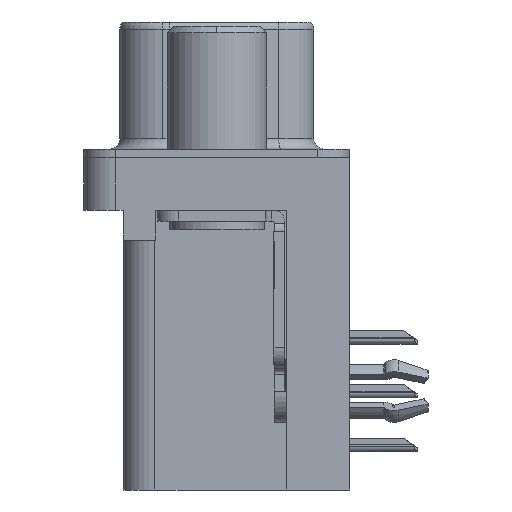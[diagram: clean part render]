
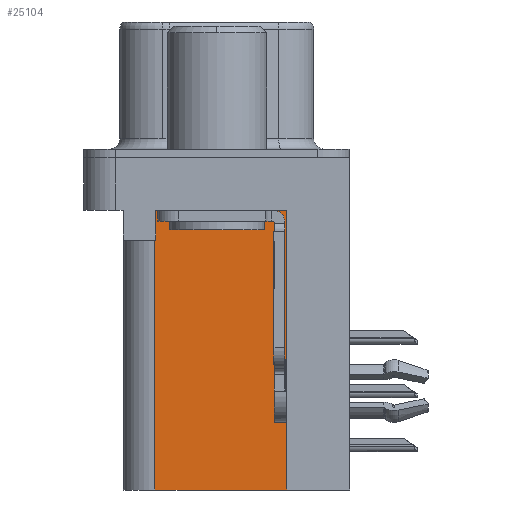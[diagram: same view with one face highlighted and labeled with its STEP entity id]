
A CAD part, left-side view. The second image highlights one B-rep face of the part: STEP entity #25104.
In plain terms, the highlighted planar face has unit normal (-1, 0, 0).
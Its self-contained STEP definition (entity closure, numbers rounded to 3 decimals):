
#221 = ORIENTED_EDGE ( 'NONE', *, *, #28423, .T. ) ;
#751 = VERTEX_POINT ( 'NONE', #20464 ) ;
#1401 = ORIENTED_EDGE ( 'NONE', *, *, #23265, .T. ) ;
#1830 = LINE ( 'NONE', #17029, #31640 ) ;
#3421 = CARTESIAN_POINT ( 'NONE',  ( 3.79, 2.925, -15.7 ) ) ;
#4382 = VERTEX_POINT ( 'NONE', #11301 ) ;
#4682 = DIRECTION ( 'NONE',  ( 0., 0., 1. ) ) ;
#5003 = VECTOR ( 'NONE', #7227, 1000. ) ;
#5517 = CARTESIAN_POINT ( 'NONE',  ( 3.79, 2.895, -3.9 ) ) ;
#5642 = DIRECTION ( 'NONE',  ( 0., 0., -1. ) ) ;
#7227 = DIRECTION ( 'NONE',  ( 0., 1., 0. ) ) ;
#8448 = VERTEX_POINT ( 'NONE', #3421 ) ;
#9052 = ORIENTED_EDGE ( 'NONE', *, *, #11153, .T. ) ;
#9829 = CARTESIAN_POINT ( 'NONE',  ( 3.79, -3.295, -2.5 ) ) ;
#9920 = VERTEX_POINT ( 'NONE', #9829 ) ;
#10063 = ORIENTED_EDGE ( 'NONE', *, *, #30349, .F. ) ;
#11153 = EDGE_CURVE ( 'NONE', #20667, #4382, #27150, .T. ) ;
#11301 = CARTESIAN_POINT ( 'NONE',  ( 3.79, 2.925, -3.9 ) ) ;
#11410 = VECTOR ( 'NONE', #4682, 1000. ) ;
#11549 = AXIS2_PLACEMENT_3D ( 'NONE', #33708, #36646, #19362 ) ;
#12090 = VECTOR ( 'NONE', #14175, 1000. ) ;
#13230 = EDGE_LOOP ( 'NONE', ( #1401, #23926, #9052, #16530, #10063, #221 ) ) ;
#13556 = PLANE ( 'NONE',  #11549 ) ;
#14175 = DIRECTION ( 'NONE',  ( 0., 0., 1. ) ) ;
#14197 = EDGE_CURVE ( 'NONE', #8448, #4382, #28330, .T. ) ;
#15445 = CARTESIAN_POINT ( 'NONE',  ( 3.79, -3.295, -2.5 ) ) ;
#16207 = CARTESIAN_POINT ( 'NONE',  ( 3.79, -3.295, -15.7 ) ) ;
#16530 = ORIENTED_EDGE ( 'NONE', *, *, #14197, .F. ) ;
#16714 = VECTOR ( 'NONE', #5642, 1000. ) ;
#17029 = CARTESIAN_POINT ( 'NONE',  ( 3.79, -3.295, -15.7 ) ) ;
#19362 = DIRECTION ( 'NONE',  ( 0., 0., -1. ) ) ;
#19970 = CARTESIAN_POINT ( 'NONE',  ( 3.79, 2.925, -15.7 ) ) ;
#20464 = CARTESIAN_POINT ( 'NONE',  ( 3.79, 2.895, -2.5 ) ) ;
#20667 = VERTEX_POINT ( 'NONE', #5517 ) ;
#22508 = FACE_OUTER_BOUND ( 'NONE', #13230, .T. ) ;
#23265 = EDGE_CURVE ( 'NONE', #9920, #751, #30709, .T. ) ;
#23926 = ORIENTED_EDGE ( 'NONE', *, *, #23981, .T. ) ;
#23981 = EDGE_CURVE ( 'NONE', #751, #20667, #32036, .T. ) ;
#24518 = VERTEX_POINT ( 'NONE', #25461 ) ;
#24527 = CARTESIAN_POINT ( 'NONE',  ( 3.79, 0., -3.9 ) ) ;
#25104 = ADVANCED_FACE ( 'NONE', ( #22508 ), #13556, .F. ) ;
#25461 = CARTESIAN_POINT ( 'NONE',  ( 3.79, -3.295, -15.7 ) ) ;
#26420 = DIRECTION ( 'NONE',  ( 0., 1., 0. ) ) ;
#27150 = LINE ( 'NONE', #24527, #5003 ) ;
#28330 = LINE ( 'NONE', #19970, #12090 ) ;
#28423 = EDGE_CURVE ( 'NONE', #24518, #9920, #34428, .T. ) ;
#30349 = EDGE_CURVE ( 'NONE', #24518, #8448, #1830, .T. ) ;
#30709 = LINE ( 'NONE', #15445, #32526 ) ;
#31640 = VECTOR ( 'NONE', #26420, 1000. ) ;
#32036 = LINE ( 'NONE', #34562, #16714 ) ;
#32526 = VECTOR ( 'NONE', #35632, 1000. ) ;
#33708 = CARTESIAN_POINT ( 'NONE',  ( 3.79, -3.295, -15.7 ) ) ;
#34428 = LINE ( 'NONE', #16207, #11410 ) ;
#34562 = CARTESIAN_POINT ( 'NONE',  ( 3.79, 2.895, -3.9 ) ) ;
#35632 = DIRECTION ( 'NONE',  ( 0., 1., 0. ) ) ;
#36646 = DIRECTION ( 'NONE',  ( 1., 0., 0. ) ) ;
